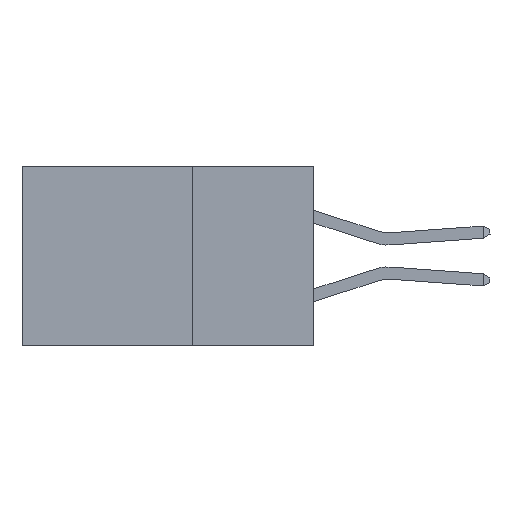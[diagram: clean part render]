
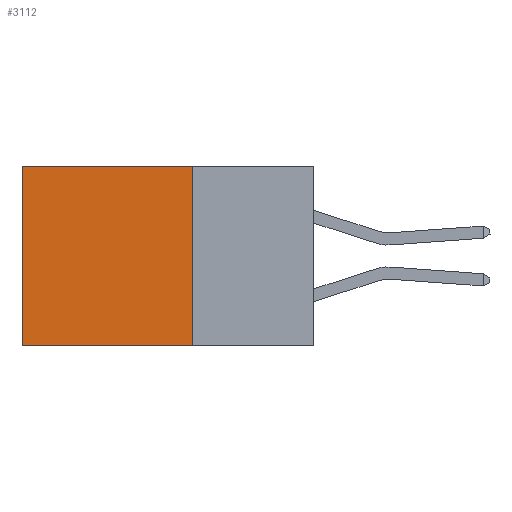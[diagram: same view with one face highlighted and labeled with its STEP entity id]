
A CAD part, left-side view. The second image highlights one B-rep face of the part: STEP entity #3112.
In plain terms, the highlighted planar face has unit normal (-1, 0, 0).
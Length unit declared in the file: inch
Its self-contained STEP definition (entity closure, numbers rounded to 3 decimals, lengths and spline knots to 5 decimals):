
#617 = LINE ( 'NONE', #3513, #10256 ) ;
#649 = CARTESIAN_POINT ( 'NONE',  ( 0.2875, 0.25, 0. ) ) ;
#1019 = DIRECTION ( 'NONE',  ( 0., 0., -1. ) ) ;
#1170 = ORIENTED_EDGE ( 'NONE', *, *, #4377, .F. ) ;
#1233 = VECTOR ( 'NONE', #5766, 39.37008 ) ;
#1990 = PLANE ( 'NONE',  #3975 ) ;
#2137 = LINE ( 'NONE', #12654, #10142 ) ;
#2803 = CARTESIAN_POINT ( 'NONE',  ( 0.2875, 0.25, 0. ) ) ;
#2998 = VERTEX_POINT ( 'NONE', #5565 ) ;
#3112 = ADVANCED_FACE ( 'NONE', ( #8984 ), #1990, .F. ) ;
#3513 = CARTESIAN_POINT ( 'NONE',  ( 0.2875, 0.6, 0. ) ) ;
#3975 = AXIS2_PLACEMENT_3D ( 'NONE', #10070, #6845, #1019 ) ;
#3977 = VERTEX_POINT ( 'NONE', #9669 ) ;
#4377 = EDGE_CURVE ( 'NONE', #11480, #10753, #2137, .T. ) ;
#4437 = CARTESIAN_POINT ( 'NONE',  ( 0.2875, 0.25, -0.37 ) ) ;
#4603 = LINE ( 'NONE', #649, #1233 ) ;
#5279 = ORIENTED_EDGE ( 'NONE', *, *, #6244, .T. ) ;
#5565 = CARTESIAN_POINT ( 'NONE',  ( 0.2875, 0.6, 0. ) ) ;
#5766 = DIRECTION ( 'NONE',  ( 0., 1., 0. ) ) ;
#5944 = VECTOR ( 'NONE', #11705, 39.37008 ) ;
#6145 = ORIENTED_EDGE ( 'NONE', *, *, #6633, .F. ) ;
#6244 = EDGE_CURVE ( 'NONE', #3977, #2998, #4603, .T. ) ;
#6633 = EDGE_CURVE ( 'NONE', #3977, #11480, #8703, .T. ) ;
#6845 = DIRECTION ( 'NONE',  ( 1., 0., 0. ) ) ;
#7039 = EDGE_LOOP ( 'NONE', ( #8282, #1170, #6145, #5279 ) ) ;
#7601 = DIRECTION ( 'NONE',  ( 0., 0., -1. ) ) ;
#8273 = EDGE_CURVE ( 'NONE', #2998, #10753, #617, .T. ) ;
#8282 = ORIENTED_EDGE ( 'NONE', *, *, #8273, .T. ) ;
#8703 = LINE ( 'NONE', #2803, #5944 ) ;
#8747 = DIRECTION ( 'NONE',  ( 0., 1., 0. ) ) ;
#8984 = FACE_OUTER_BOUND ( 'NONE', #7039, .T. ) ;
#9669 = CARTESIAN_POINT ( 'NONE',  ( 0.2875, 0.25, 0. ) ) ;
#10070 = CARTESIAN_POINT ( 'NONE',  ( 0.2875, 0.25, 0. ) ) ;
#10142 = VECTOR ( 'NONE', #8747, 39.37008 ) ;
#10256 = VECTOR ( 'NONE', #7601, 39.37008 ) ;
#10753 = VERTEX_POINT ( 'NONE', #10765 ) ;
#10765 = CARTESIAN_POINT ( 'NONE',  ( 0.2875, 0.6, -0.37 ) ) ;
#11480 = VERTEX_POINT ( 'NONE', #4437 ) ;
#11705 = DIRECTION ( 'NONE',  ( 0., 0., -1. ) ) ;
#12654 = CARTESIAN_POINT ( 'NONE',  ( 0.2875, 0.25, -0.37 ) ) ;
